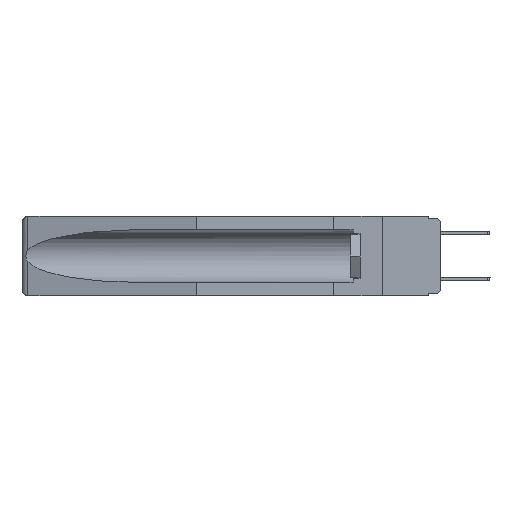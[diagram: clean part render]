
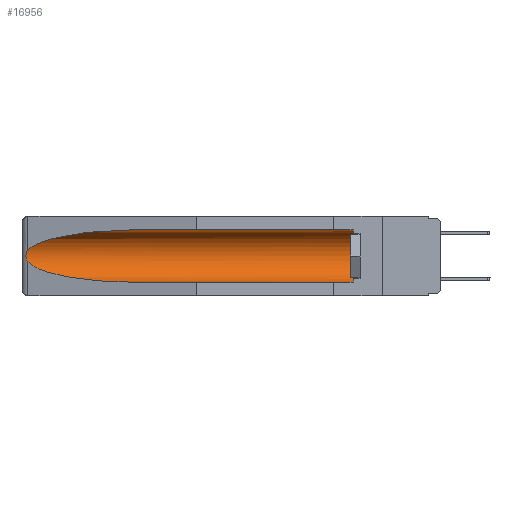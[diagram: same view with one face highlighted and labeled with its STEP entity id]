
A CAD part, left-side view. The second image highlights one B-rep face of the part: STEP entity #16956.
In plain terms, the highlighted cylindrical face has radius 2.857 mm (diameter 5.715 mm), a partial arc.
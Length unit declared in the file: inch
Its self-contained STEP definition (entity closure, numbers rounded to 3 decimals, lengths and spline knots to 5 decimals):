
#19 = EDGE_CURVE ( 'NONE', #12176, #14134, #8363, .T. ) ;
#91 = CARTESIAN_POINT ( 'NONE',  ( 0.2673, 1.53269, -0.17917 ) ) ;
#200 = CARTESIAN_POINT ( 'NONE',  ( 0.155, -0.30754, -0.284 ) ) ;
#790 = DIRECTION ( 'NONE',  ( 0., 1., 0. ) ) ;
#990 = CARTESIAN_POINT ( 'NONE',  ( 0.155, -0.30754, -0.1715 ) ) ;
#1297 = DIRECTION ( 'NONE',  ( 0., -1., 0. ) ) ;
#1391 = CARTESIAN_POINT ( 'NONE',  ( 0.155, 0.126, -0.284 ) ) ;
#1592 = CARTESIAN_POINT ( 'NONE',  ( 0.26597, 1.5296, -0.19026 ) ) ;
#2162 = CARTESIAN_POINT ( 'NONE',  ( 0.21114, 1.30732, -0.284 ) ) ;
#2518 = CARTESIAN_POINT ( 'NONE',  ( 0.26537, 1.52718, -0.14972 ) ) ;
#2830 = CARTESIAN_POINT ( 'NONE',  ( 0.26655, 1.53094, -0.18657 ) ) ;
#2903 = CARTESIAN_POINT ( 'NONE',  ( 0.2675, 1.53308, -0.17534 ) ) ;
#3891 = VECTOR ( 'NONE', #790, 39.37008 ) ;
#4156 = CARTESIAN_POINT ( 'NONE',  ( 0.26537, 1.52718, -0.14972 ) ) ;
#4170 = CARTESIAN_POINT ( 'NONE',  ( 0.155, 1.07973, -0.284 ) ) ;
#4549 = CARTESIAN_POINT ( 'NONE',  ( 0.26537, 1.52718, -0.19328 ) ) ;
#5024 = CARTESIAN_POINT ( 'NONE',  ( 0.21114, 1.30732, -0.059 ) ) ;
#5214 = EDGE_CURVE ( 'NONE', #12176, #11847, #10947, .T. ) ;
#5437 = ORIENTED_EDGE ( 'NONE', *, *, #11250, .T. ) ;
#5544 = CARTESIAN_POINT ( 'NONE',  ( 0.2673, 1.5327, -0.16383 ) ) ;
#5551 = LINE ( 'NONE', #16470, #3891 ) ;
#5733 = DIRECTION ( 'NONE',  ( 0., 1., 0. ) ) ;
#6062 = AXIS2_PLACEMENT_3D ( 'NONE', #9360, #1297, #13565 ) ;
#6525 = CARTESIAN_POINT ( 'NONE',  ( 0.26537, 1.52718, -0.14972 ) ) ;
#6680 = B_SPLINE_CURVE_WITH_KNOTS ( 'NONE', 3,
 ( #4156, #9587, #10839, #5544, #13864, #2903, #91, #2830, #1592, #9837 ),
 .UNSPECIFIED., .F., .F.,
 ( 4, 2, 2, 2, 4 ),
 ( 0., 0.00029, 0.00058, 0.00087, 0.00117 ),
 .UNSPECIFIED. ) ;
#7426 = FACE_OUTER_BOUND ( 'NONE', #10549, .T. ) ;
#7799 = CARTESIAN_POINT ( 'NONE',  ( 0.25451, 1.48313, -0.09465 ) ) ;
#7896 = CARTESIAN_POINT ( 'NONE',  ( 0.155, 1.07973, -0.059 ) ) ;
#8201 = EDGE_CURVE ( 'NONE', #9635, #14134, #17479, .T. ) ;
#8363 = LINE ( 'NONE', #200, #13370 ) ;
#9116 = ORIENTED_EDGE ( 'NONE', *, *, #11155, .T. ) ;
#9360 = CARTESIAN_POINT ( 'NONE',  ( 0.155, 0.126, -0.1715 ) ) ;
#9513 =( BOUNDED_CURVE ( )  B_SPLINE_CURVE ( 3, ( #7896, #5024, #7799, #6525 ),
 .UNSPECIFIED., .F., .T. ) 
 B_SPLINE_CURVE_WITH_KNOTS ( ( 4, 4 ),
 ( 4.71239, 6.08839 ),
 .UNSPECIFIED. ) 
 CURVE ( )  GEOMETRIC_REPRESENTATION_ITEM ( )  RATIONAL_B_SPLINE_CURVE ( ( 1., 0.848, 0.848, 1. ) ) 
 REPRESENTATION_ITEM ( '' )  );
#9587 = CARTESIAN_POINT ( 'NONE',  ( 0.26597, 1.52961, -0.15275 ) ) ;
#9635 = VERTEX_POINT ( 'NONE', #15123 ) ;
#9837 = CARTESIAN_POINT ( 'NONE',  ( 0.26537, 1.52718, -0.19328 ) ) ;
#9965 = ORIENTED_EDGE ( 'NONE', *, *, #17240, .T. ) ;
#10167 = CARTESIAN_POINT ( 'NONE',  ( 0.155, 0.126, -0.059 ) ) ;
#10549 = EDGE_LOOP ( 'NONE', ( #9116, #5437, #11614, #11982, #12258, #9965 ) ) ;
#10839 = CARTESIAN_POINT ( 'NONE',  ( 0.26654, 1.53092, -0.15636 ) ) ;
#10947 = CIRCLE ( 'NONE', #6062, 0.1125 ) ;
#11155 = EDGE_CURVE ( 'NONE', #12160, #11968, #9513, .T. ) ;
#11250 = EDGE_CURVE ( 'NONE', #11968, #9635, #6680, .T. ) ;
#11388 = DIRECTION ( 'NONE',  ( 0., 1., 0. ) ) ;
#11511 = CARTESIAN_POINT ( 'NONE',  ( 0.25451, 1.48313, -0.24835 ) ) ;
#11614 = ORIENTED_EDGE ( 'NONE', *, *, #8201, .T. ) ;
#11847 = VERTEX_POINT ( 'NONE', #10167 ) ;
#11968 = VERTEX_POINT ( 'NONE', #2518 ) ;
#11982 = ORIENTED_EDGE ( 'NONE', *, *, #19, .F. ) ;
#12160 = VERTEX_POINT ( 'NONE', #17569 ) ;
#12176 = VERTEX_POINT ( 'NONE', #1391 ) ;
#12258 = ORIENTED_EDGE ( 'NONE', *, *, #5214, .T. ) ;
#13370 = VECTOR ( 'NONE', #5733, 39.37008 ) ;
#13565 = DIRECTION ( 'NONE',  ( 0., 0., 1. ) ) ;
#13864 = CARTESIAN_POINT ( 'NONE',  ( 0.2675, 1.53308, -0.16763 ) ) ;
#14134 = VERTEX_POINT ( 'NONE', #4170 ) ;
#14269 = CARTESIAN_POINT ( 'NONE',  ( 0.155, 1.07973, -0.284 ) ) ;
#14403 = CYLINDRICAL_SURFACE ( 'NONE', #15526, 0.1125 ) ;
#15123 = CARTESIAN_POINT ( 'NONE',  ( 0.26537, 1.52718, -0.19328 ) ) ;
#15480 = DIRECTION ( 'NONE',  ( 0., 0., 1. ) ) ;
#15526 = AXIS2_PLACEMENT_3D ( 'NONE', #990, #11388, #15480 ) ;
#16470 = CARTESIAN_POINT ( 'NONE',  ( 0.155, -0.30754, -0.059 ) ) ;
#16956 = ADVANCED_FACE ( 'NONE', ( #7426 ), #14403, .F. ) ;
#17240 = EDGE_CURVE ( 'NONE', #11847, #12160, #5551, .T. ) ;
#17479 =( BOUNDED_CURVE ( )  B_SPLINE_CURVE ( 3, ( #4549, #11511, #2162, #14269 ),
 .UNSPECIFIED., .F., .T. ) 
 B_SPLINE_CURVE_WITH_KNOTS ( ( 4, 4 ),
 ( 0.1948, 1.5708 ),
 .UNSPECIFIED. ) 
 CURVE ( )  GEOMETRIC_REPRESENTATION_ITEM ( )  RATIONAL_B_SPLINE_CURVE ( ( 1., 0.848, 0.848, 1. ) ) 
 REPRESENTATION_ITEM ( '' )  );
#17569 = CARTESIAN_POINT ( 'NONE',  ( 0.155, 1.07973, -0.059 ) ) ;
